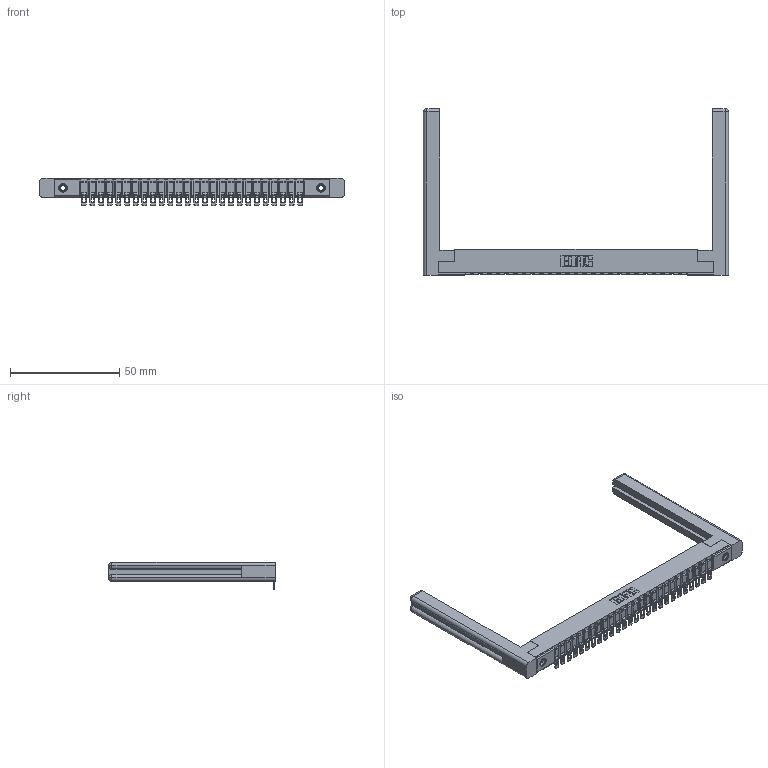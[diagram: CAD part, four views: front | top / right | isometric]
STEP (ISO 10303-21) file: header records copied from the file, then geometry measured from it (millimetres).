
FILE_DESCRIPTION (( 'STEP AP203' ), '1' );
FILE_NAME ('307-026-554-158.STEP', '2019-09-05T02:14:25', ( '' ), ( '' ), 'SwSTEP 2.0', 'SolidWorks 2016', '' );
FILE_SCHEMA (( 'CONFIG_CONTROL_DESIGN' ));
Length unit declared in the file: inch
Products named in the file (5): 307-026-554-158; 307 Part_.156 Dia Mounting Holes; 345-250-001_345-250-001-102; 307-220-058; 307-290-002_554
Assembly tree (31 placements, depth 2):
  307-026-554-158
    307 Part_.156 Dia Mounting Holes
    307-290-002_554  x26
    307-220-058  x2
    345-250-001_345-250-001-102  x2
Bounding box: 139.65 x 76.33 x 12.52 mm (x, y, z)
Volume: 16909.2 mm3; surface area: 22143.1 mm2
Topology: 31 solids, 31 shells, 2393 faces, 7255 edges, 4750 vertices
Faces by surface type: plane 1350, cylinder 965, sphere 54, torus 12, cone 12
Entity records: 27860 total; most frequent: CARTESIAN_POINT 4705, ORIENTED_EDGE 4634, DIRECTION 4545, EDGE_CURVE 2317, LINE 1757, VECTOR 1757, VERTEX_POINT 1500, AXIS2_PLACEMENT_3D 1394
